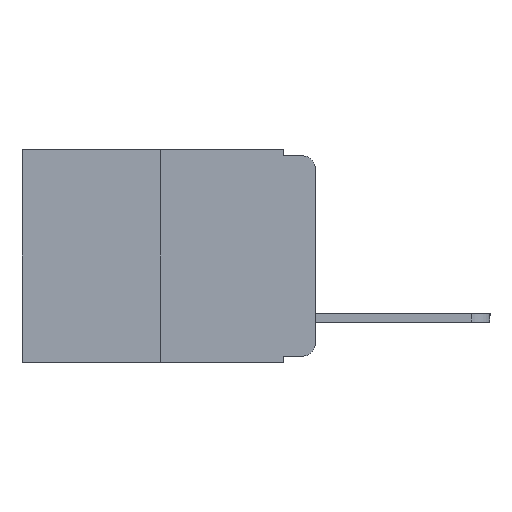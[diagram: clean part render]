
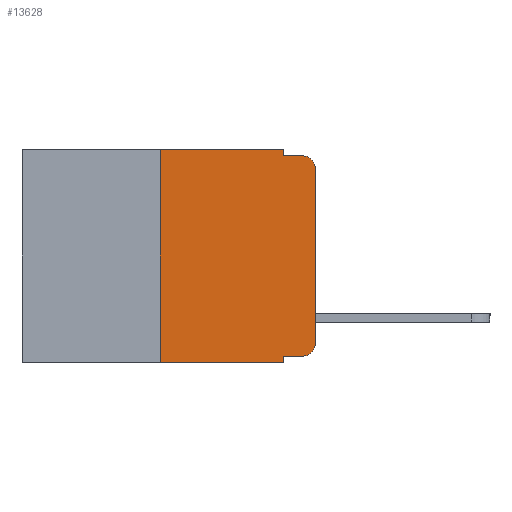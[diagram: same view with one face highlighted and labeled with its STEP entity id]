
A CAD part, left-side view. The second image highlights one B-rep face of the part: STEP entity #13628.
In plain terms, the highlighted planar face has unit normal (-1, 0, 0).
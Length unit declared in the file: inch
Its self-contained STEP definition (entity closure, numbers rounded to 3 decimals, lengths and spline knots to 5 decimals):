
#88 = ORIENTED_EDGE ( 'NONE', *, *, #13212, .T. ) ;
#267 = CARTESIAN_POINT ( 'NONE',  ( 0., 0.051, -0.01 ) ) ;
#363 = CARTESIAN_POINT ( 'NONE',  ( 0., 0.25, -0.343 ) ) ;
#378 = EDGE_CURVE ( 'NONE', #9567, #6568, #17581, .T. ) ;
#564 = LINE ( 'NONE', #267, #4317 ) ;
#646 = PLANE ( 'NONE',  #13661 ) ;
#647 = ORIENTED_EDGE ( 'NONE', *, *, #18289, .F. ) ;
#808 = VERTEX_POINT ( 'NONE', #3774 ) ;
#927 = DIRECTION ( 'NONE',  ( -1., 0., 0. ) ) ;
#968 = CARTESIAN_POINT ( 'NONE',  ( 0., 0.051, 0. ) ) ;
#1149 = DIRECTION ( 'NONE',  ( 0., 0., -1. ) ) ;
#1576 = VECTOR ( 'NONE', #1748, 39.37008 ) ;
#1580 = LINE ( 'NONE', #13684, #9405 ) ;
#1744 = DIRECTION ( 'NONE',  ( 0., -1., 0. ) ) ;
#1748 = DIRECTION ( 'NONE',  ( 0., -1., 0. ) ) ;
#1772 = CARTESIAN_POINT ( 'NONE',  ( 0., 0.473, -0.343 ) ) ;
#2199 = VECTOR ( 'NONE', #3895, 39.37008 ) ;
#2436 = VERTEX_POINT ( 'NONE', #5851 ) ;
#2457 = CARTESIAN_POINT ( 'NONE',  ( 0., 0.25, 0. ) ) ;
#2689 = VECTOR ( 'NONE', #1744, 39.37008 ) ;
#2737 = EDGE_CURVE ( 'NONE', #8215, #6568, #17760, .T. ) ;
#3163 = CIRCLE ( 'NONE', #12600, 0.02 ) ;
#3669 = VERTEX_POINT ( 'NONE', #968 ) ;
#3774 = CARTESIAN_POINT ( 'NONE',  ( 0., 0.02, -0.01 ) ) ;
#3895 = DIRECTION ( 'NONE',  ( 0., 0., 1. ) ) ;
#4131 = ORIENTED_EDGE ( 'NONE', *, *, #9093, .T. ) ;
#4217 = DIRECTION ( 'NONE',  ( -1., 0., 0. ) ) ;
#4317 = VECTOR ( 'NONE', #17438, 39.37008 ) ;
#4552 = AXIS2_PLACEMENT_3D ( 'NONE', #10288, #927, #11828 ) ;
#4693 = CARTESIAN_POINT ( 'NONE',  ( 0., 0.051, 0. ) ) ;
#4957 = VECTOR ( 'NONE', #17810, 39.37008 ) ;
#5191 = EDGE_CURVE ( 'NONE', #9567, #13283, #19557, .T. ) ;
#5517 = VECTOR ( 'NONE', #1149, 39.37008 ) ;
#5851 = CARTESIAN_POINT ( 'NONE',  ( 0., 0.02, -0.333 ) ) ;
#6259 = FACE_OUTER_BOUND ( 'NONE', #14253, .T. ) ;
#6568 = VERTEX_POINT ( 'NONE', #7091 ) ;
#6932 = DIRECTION ( 'NONE',  ( 0., 0., -1. ) ) ;
#6973 = ORIENTED_EDGE ( 'NONE', *, *, #17996, .F. ) ;
#7091 = CARTESIAN_POINT ( 'NONE',  ( 0., 0.051, -0.343 ) ) ;
#7151 = ORIENTED_EDGE ( 'NONE', *, *, #7234, .T. ) ;
#7234 = EDGE_CURVE ( 'NONE', #2436, #8301, #19369, .T. ) ;
#8215 = VERTEX_POINT ( 'NONE', #17211 ) ;
#8301 = VERTEX_POINT ( 'NONE', #18941 ) ;
#8859 = ORIENTED_EDGE ( 'NONE', *, *, #18648, .T. ) ;
#9093 = EDGE_CURVE ( 'NONE', #17932, #808, #3163, .T. ) ;
#9405 = VECTOR ( 'NONE', #15249, 39.37008 ) ;
#9567 = VERTEX_POINT ( 'NONE', #363 ) ;
#9583 = ORIENTED_EDGE ( 'NONE', *, *, #2737, .F. ) ;
#9671 = LINE ( 'NONE', #19698, #5517 ) ;
#9977 = CARTESIAN_POINT ( 'NONE',  ( 0., 0., 0. ) ) ;
#10034 = CARTESIAN_POINT ( 'NONE',  ( 0., 0.473, 0. ) ) ;
#10288 = CARTESIAN_POINT ( 'NONE',  ( 0., 0.02, -0.313 ) ) ;
#10438 = CARTESIAN_POINT ( 'NONE',  ( 0., 0.051, -0.01 ) ) ;
#11828 = DIRECTION ( 'NONE',  ( 0., 0., -1. ) ) ;
#12600 = AXIS2_PLACEMENT_3D ( 'NONE', #13446, #4217, #14995 ) ;
#13212 = EDGE_CURVE ( 'NONE', #8301, #17932, #14520, .T. ) ;
#13283 = VERTEX_POINT ( 'NONE', #2457 ) ;
#13366 = VERTEX_POINT ( 'NONE', #10438 ) ;
#13446 = CARTESIAN_POINT ( 'NONE',  ( 0., 0.02, -0.03 ) ) ;
#13454 = CARTESIAN_POINT ( 'NONE',  ( 0., 0., -0.03 ) ) ;
#13628 = ADVANCED_FACE ( 'NONE', ( #6259 ), #646, .F. ) ;
#13661 = AXIS2_PLACEMENT_3D ( 'NONE', #10034, #16236, #6932 ) ;
#13684 = CARTESIAN_POINT ( 'NONE',  ( 0., 0.051, -0.333 ) ) ;
#14119 = ORIENTED_EDGE ( 'NONE', *, *, #5191, .F. ) ;
#14253 = EDGE_LOOP ( 'NONE', ( #88, #4131, #647, #6973, #15794, #14119, #14859, #9583, #8859, #7151 ) ) ;
#14516 = LINE ( 'NONE', #17193, #2689 ) ;
#14520 = LINE ( 'NONE', #9977, #2199 ) ;
#14859 = ORIENTED_EDGE ( 'NONE', *, *, #378, .T. ) ;
#14995 = DIRECTION ( 'NONE',  ( 0., 0., -1. ) ) ;
#15249 = DIRECTION ( 'NONE',  ( 0., -1., 0. ) ) ;
#15468 = VECTOR ( 'NONE', #18042, 39.37008 ) ;
#15794 = ORIENTED_EDGE ( 'NONE', *, *, #15818, .F. ) ;
#15818 = EDGE_CURVE ( 'NONE', #13283, #3669, #14516, .T. ) ;
#16236 = DIRECTION ( 'NONE',  ( 1., 0., 0. ) ) ;
#17193 = CARTESIAN_POINT ( 'NONE',  ( 0., 0.473, 0. ) ) ;
#17211 = CARTESIAN_POINT ( 'NONE',  ( 0., 0.051, -0.333 ) ) ;
#17438 = DIRECTION ( 'NONE',  ( 0., -1., 0. ) ) ;
#17581 = LINE ( 'NONE', #1772, #1576 ) ;
#17760 = LINE ( 'NONE', #4693, #4957 ) ;
#17810 = DIRECTION ( 'NONE',  ( 0., 0., -1. ) ) ;
#17932 = VERTEX_POINT ( 'NONE', #13454 ) ;
#17996 = EDGE_CURVE ( 'NONE', #3669, #13366, #9671, .T. ) ;
#18042 = DIRECTION ( 'NONE',  ( 0., 0., 1. ) ) ;
#18289 = EDGE_CURVE ( 'NONE', #13366, #808, #564, .T. ) ;
#18648 = EDGE_CURVE ( 'NONE', #8215, #2436, #1580, .T. ) ;
#18941 = CARTESIAN_POINT ( 'NONE',  ( 0., 0., -0.313 ) ) ;
#19369 = CIRCLE ( 'NONE', #4552, 0.02 ) ;
#19557 = LINE ( 'NONE', #19572, #15468 ) ;
#19572 = CARTESIAN_POINT ( 'NONE',  ( 0., 0.25, 0. ) ) ;
#19698 = CARTESIAN_POINT ( 'NONE',  ( 0., 0.051, 0. ) ) ;
